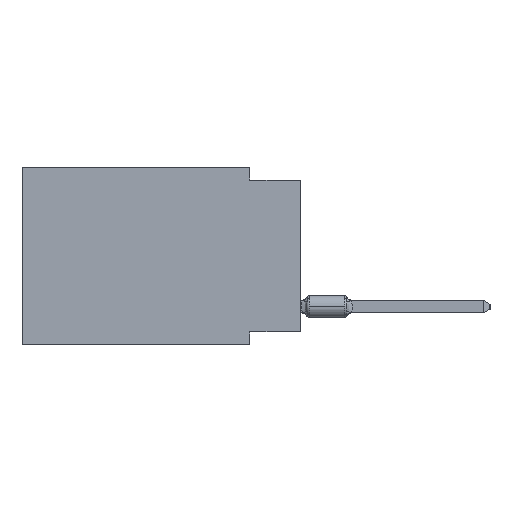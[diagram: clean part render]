
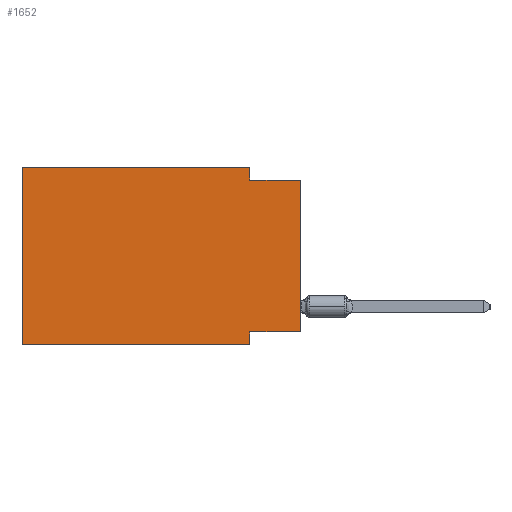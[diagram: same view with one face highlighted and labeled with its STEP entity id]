
A CAD part, left-side view. The second image highlights one B-rep face of the part: STEP entity #1652.
In plain terms, the highlighted planar face has unit normal (-1, 0, 0).
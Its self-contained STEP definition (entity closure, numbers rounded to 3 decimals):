
#1622 = LINE ( 'NONE', #12546, #39863 ) ;
#1652 = ADVANCED_FACE ( 'NONE', ( #12673 ), #23530, .F. ) ;
#2194 = VECTOR ( 'NONE', #42960, 1000. ) ;
#4086 = VECTOR ( 'NONE', #5429, 1000. ) ;
#4651 = EDGE_LOOP ( 'NONE', ( #29998, #27732, #20607, #11379, #35211, #23737, #28035, #24043 ) ) ;
#4730 = DIRECTION ( 'NONE',  ( 0., 0., -1. ) ) ;
#4779 = EDGE_CURVE ( 'NONE', #24108, #41189, #9329, .T. ) ;
#4914 = LINE ( 'NONE', #45781, #41116 ) ;
#4927 = LINE ( 'NONE', #35389, #4086 ) ;
#5108 = CARTESIAN_POINT ( 'NONE',  ( 0., 2.54, 0. ) ) ;
#5128 = CARTESIAN_POINT ( 'NONE',  ( 0., 2.54, -8.255 ) ) ;
#5429 = DIRECTION ( 'NONE',  ( 0., 0., 1. ) ) ;
#7583 = AXIS2_PLACEMENT_3D ( 'NONE', #8931, #11669, #4730 ) ;
#8199 = CARTESIAN_POINT ( 'NONE',  ( 0., 13.97, -8.89 ) ) ;
#8931 = CARTESIAN_POINT ( 'NONE',  ( 0., 13.97, 0. ) ) ;
#9329 = LINE ( 'NONE', #5108, #42704 ) ;
#11379 = ORIENTED_EDGE ( 'NONE', *, *, #17362, .F. ) ;
#11669 = DIRECTION ( 'NONE',  ( 1., 0., 0. ) ) ;
#11881 = EDGE_CURVE ( 'NONE', #44428, #20374, #4914, .T. ) ;
#12546 = CARTESIAN_POINT ( 'NONE',  ( 0., 2.54, -8.89 ) ) ;
#12673 = FACE_OUTER_BOUND ( 'NONE', #4651, .T. ) ;
#14316 = CARTESIAN_POINT ( 'NONE',  ( 0., 2.54, -0.635 ) ) ;
#16713 = LINE ( 'NONE', #35026, #2194 ) ;
#17362 = EDGE_CURVE ( 'NONE', #42976, #24108, #16713, .T. ) ;
#18743 = CARTESIAN_POINT ( 'NONE',  ( 0., 13.97, 0. ) ) ;
#20374 = VERTEX_POINT ( 'NONE', #5128 ) ;
#20460 = DIRECTION ( 'NONE',  ( 0., 0., -1. ) ) ;
#20607 = ORIENTED_EDGE ( 'NONE', *, *, #4779, .F. ) ;
#21817 = LINE ( 'NONE', #45573, #29649 ) ;
#22518 = VERTEX_POINT ( 'NONE', #29017 ) ;
#23530 = PLANE ( 'NONE',  #7583 ) ;
#23551 = DIRECTION ( 'NONE',  ( 0., -1., 0. ) ) ;
#23737 = ORIENTED_EDGE ( 'NONE', *, *, #23771, .T. ) ;
#23771 = EDGE_CURVE ( 'NONE', #22518, #47370, #27026, .T. ) ;
#24043 = ORIENTED_EDGE ( 'NONE', *, *, #11881, .F. ) ;
#24108 = VERTEX_POINT ( 'NONE', #31626 ) ;
#26119 = CARTESIAN_POINT ( 'NONE',  ( 0., 0., -0.635 ) ) ;
#27026 = LINE ( 'NONE', #8199, #39827 ) ;
#27732 = ORIENTED_EDGE ( 'NONE', *, *, #33801, .F. ) ;
#28035 = ORIENTED_EDGE ( 'NONE', *, *, #35934, .F. ) ;
#29017 = CARTESIAN_POINT ( 'NONE',  ( 0., 13.97, -8.89 ) ) ;
#29649 = VECTOR ( 'NONE', #41367, 1000. ) ;
#29998 = ORIENTED_EDGE ( 'NONE', *, *, #47169, .T. ) ;
#31626 = CARTESIAN_POINT ( 'NONE',  ( 0., 2.54, 0. ) ) ;
#33615 = EDGE_CURVE ( 'NONE', #22518, #42976, #4927, .T. ) ;
#33801 = EDGE_CURVE ( 'NONE', #41189, #41967, #37291, .T. ) ;
#34145 = DIRECTION ( 'NONE',  ( 0., 1., 0. ) ) ;
#35026 = CARTESIAN_POINT ( 'NONE',  ( 0., 13.97, 0. ) ) ;
#35211 = ORIENTED_EDGE ( 'NONE', *, *, #33615, .F. ) ;
#35389 = CARTESIAN_POINT ( 'NONE',  ( 0., 13.97, 0. ) ) ;
#35934 = EDGE_CURVE ( 'NONE', #20374, #47370, #1622, .T. ) ;
#37291 = LINE ( 'NONE', #26119, #37337 ) ;
#37337 = VECTOR ( 'NONE', #41237, 1000. ) ;
#39521 = DIRECTION ( 'NONE',  ( 0., 0., -1. ) ) ;
#39827 = VECTOR ( 'NONE', #23551, 1000. ) ;
#39863 = VECTOR ( 'NONE', #39521, 1000. ) ;
#41116 = VECTOR ( 'NONE', #34145, 1000. ) ;
#41189 = VERTEX_POINT ( 'NONE', #14316 ) ;
#41237 = DIRECTION ( 'NONE',  ( 0., -1., 0. ) ) ;
#41367 = DIRECTION ( 'NONE',  ( 0., 0., 1. ) ) ;
#41967 = VERTEX_POINT ( 'NONE', #45450 ) ;
#42356 = CARTESIAN_POINT ( 'NONE',  ( 0., 2.54, -8.89 ) ) ;
#42704 = VECTOR ( 'NONE', #20460, 1000. ) ;
#42960 = DIRECTION ( 'NONE',  ( 0., -1., 0. ) ) ;
#42976 = VERTEX_POINT ( 'NONE', #18743 ) ;
#43973 = CARTESIAN_POINT ( 'NONE',  ( 0., 0., -8.255 ) ) ;
#44428 = VERTEX_POINT ( 'NONE', #43973 ) ;
#45450 = CARTESIAN_POINT ( 'NONE',  ( 0., 0., -0.635 ) ) ;
#45573 = CARTESIAN_POINT ( 'NONE',  ( 0., 0., 0. ) ) ;
#45781 = CARTESIAN_POINT ( 'NONE',  ( 0., 0., -8.255 ) ) ;
#47169 = EDGE_CURVE ( 'NONE', #44428, #41967, #21817, .T. ) ;
#47370 = VERTEX_POINT ( 'NONE', #42356 ) ;
